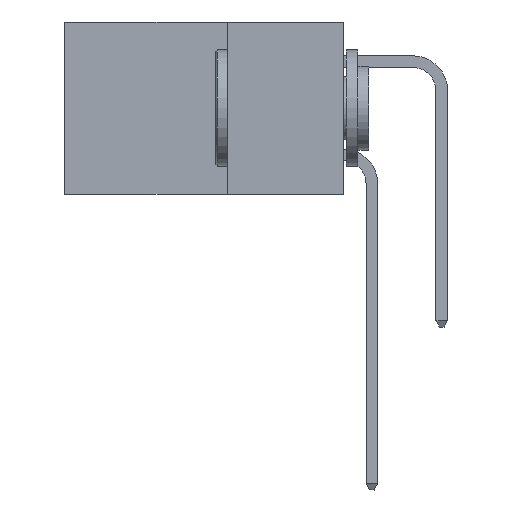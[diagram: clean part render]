
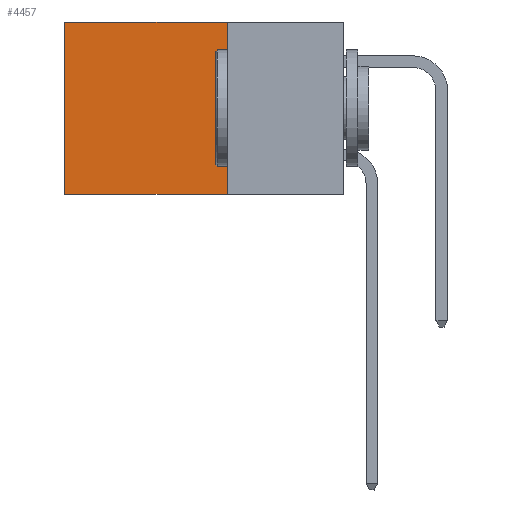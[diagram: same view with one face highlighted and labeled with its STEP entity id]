
A CAD part, left-side view. The second image highlights one B-rep face of the part: STEP entity #4457.
In plain terms, the highlighted planar face has unit normal (-1, 0, 0).
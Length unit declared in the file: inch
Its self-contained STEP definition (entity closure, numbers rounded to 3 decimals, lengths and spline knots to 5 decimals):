
#710 = FACE_OUTER_BOUND ( 'NONE', #11590, .T. ) ;
#750 = EDGE_CURVE ( 'NONE', #15592, #3441, #7600, .T. ) ;
#1128 = VERTEX_POINT ( 'NONE', #3150 ) ;
#1413 = VERTEX_POINT ( 'NONE', #12041 ) ;
#2465 = CARTESIAN_POINT ( 'NONE',  ( 0.298, 0.25, -0.37 ) ) ;
#2821 = AXIS2_PLACEMENT_3D ( 'NONE', #11074, #8722, #3466 ) ;
#3052 = LINE ( 'NONE', #11845, #4420 ) ;
#3150 = CARTESIAN_POINT ( 'NONE',  ( 0.298, 0.25, -0.37 ) ) ;
#3441 = VERTEX_POINT ( 'NONE', #9055 ) ;
#3466 = DIRECTION ( 'NONE',  ( 0., 0., -1. ) ) ;
#4420 = VECTOR ( 'NONE', #9669, 39.37008 ) ;
#4457 = ADVANCED_FACE ( 'NONE', ( #710 ), #13630, .F. ) ;
#5047 = VECTOR ( 'NONE', #6064, 39.37008 ) ;
#5110 = EDGE_CURVE ( 'NONE', #1413, #1128, #6401, .T. ) ;
#6048 = ORIENTED_EDGE ( 'NONE', *, *, #750, .T. ) ;
#6064 = DIRECTION ( 'NONE',  ( 0., 1., 0. ) ) ;
#6401 = LINE ( 'NONE', #15685, #9401 ) ;
#7118 = ORIENTED_EDGE ( 'NONE', *, *, #5110, .F. ) ;
#7600 = LINE ( 'NONE', #15711, #12898 ) ;
#8196 = DIRECTION ( 'NONE',  ( 0., 0., -1. ) ) ;
#8722 = DIRECTION ( 'NONE',  ( 1., 0., 0. ) ) ;
#9055 = CARTESIAN_POINT ( 'NONE',  ( 0.298, 0.6, -0.37 ) ) ;
#9401 = VECTOR ( 'NONE', #8196, 39.37008 ) ;
#9669 = DIRECTION ( 'NONE',  ( 0., 1., 0. ) ) ;
#10732 = DIRECTION ( 'NONE',  ( 0., 0., -1. ) ) ;
#10776 = EDGE_CURVE ( 'NONE', #1128, #3441, #15514, .T. ) ;
#11074 = CARTESIAN_POINT ( 'NONE',  ( 0.298, 0.25, 0. ) ) ;
#11590 = EDGE_LOOP ( 'NONE', ( #6048, #14838, #7118, #12752 ) ) ;
#11845 = CARTESIAN_POINT ( 'NONE',  ( 0.298, 0.25, 0. ) ) ;
#12041 = CARTESIAN_POINT ( 'NONE',  ( 0.298, 0.25, 0. ) ) ;
#12286 = EDGE_CURVE ( 'NONE', #1413, #15592, #3052, .T. ) ;
#12752 = ORIENTED_EDGE ( 'NONE', *, *, #12286, .T. ) ;
#12898 = VECTOR ( 'NONE', #10732, 39.37008 ) ;
#13630 = PLANE ( 'NONE',  #2821 ) ;
#14838 = ORIENTED_EDGE ( 'NONE', *, *, #10776, .F. ) ;
#15029 = CARTESIAN_POINT ( 'NONE',  ( 0.298, 0.6, 0. ) ) ;
#15514 = LINE ( 'NONE', #2465, #5047 ) ;
#15592 = VERTEX_POINT ( 'NONE', #15029 ) ;
#15685 = CARTESIAN_POINT ( 'NONE',  ( 0.298, 0.25, 0. ) ) ;
#15711 = CARTESIAN_POINT ( 'NONE',  ( 0.298, 0.6, 0. ) ) ;
